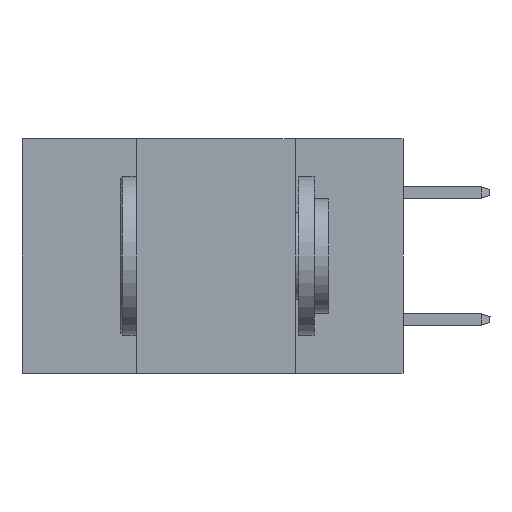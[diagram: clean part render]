
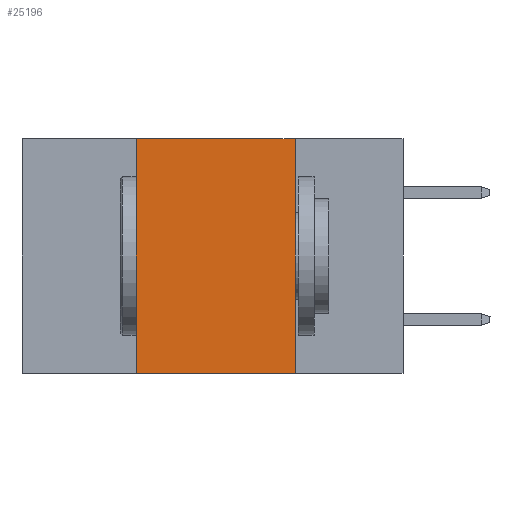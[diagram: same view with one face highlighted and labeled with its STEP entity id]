
A CAD part, left-side view. The second image highlights one B-rep face of the part: STEP entity #25196.
In plain terms, the highlighted planar face has unit normal (-1, 0, 0).
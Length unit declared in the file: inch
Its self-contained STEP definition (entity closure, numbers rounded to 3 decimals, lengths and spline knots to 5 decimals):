
#1171 = FACE_OUTER_BOUND ( 'NONE', #2502, .T. ) ;
#1726 = CARTESIAN_POINT ( 'NONE',  ( 0., 0.17, 0. ) ) ;
#1847 = DIRECTION ( 'NONE',  ( 0., -1., 0. ) ) ;
#2243 = VECTOR ( 'NONE', #7928, 39.37008 ) ;
#2502 = EDGE_LOOP ( 'NONE', ( #14716, #17885, #12714, #3835 ) ) ;
#3537 = VECTOR ( 'NONE', #1847, 39.37008 ) ;
#3766 = LINE ( 'NONE', #11602, #3537 ) ;
#3835 = ORIENTED_EDGE ( 'NONE', *, *, #11018, .T. ) ;
#4919 = VECTOR ( 'NONE', #22221, 39.37008 ) ;
#6716 = CARTESIAN_POINT ( 'NONE',  ( 0., 0.6, 0. ) ) ;
#7212 = CARTESIAN_POINT ( 'NONE',  ( 0., 0.42, -0.37 ) ) ;
#7320 = DIRECTION ( 'NONE',  ( 0., 0., -1. ) ) ;
#7928 = DIRECTION ( 'NONE',  ( 0., -1., 0. ) ) ;
#9028 = PLANE ( 'NONE',  #9874 ) ;
#9387 = CARTESIAN_POINT ( 'NONE',  ( 0., 0.17, 0. ) ) ;
#9874 = AXIS2_PLACEMENT_3D ( 'NONE', #6716, #16828, #24701 ) ;
#9923 = LINE ( 'NONE', #23919, #4919 ) ;
#11018 = EDGE_CURVE ( 'NONE', #14980, #21601, #23480, .T. ) ;
#11602 = CARTESIAN_POINT ( 'NONE',  ( 0., 0.6, 0. ) ) ;
#12053 = EDGE_CURVE ( 'NONE', #21912, #21601, #15380, .T. ) ;
#12714 = ORIENTED_EDGE ( 'NONE', *, *, #24049, .F. ) ;
#14544 = VECTOR ( 'NONE', #7320, 39.37008 ) ;
#14716 = ORIENTED_EDGE ( 'NONE', *, *, #12053, .F. ) ;
#14980 = VERTEX_POINT ( 'NONE', #7212 ) ;
#15158 = VERTEX_POINT ( 'NONE', #21239 ) ;
#15380 = LINE ( 'NONE', #9387, #14544 ) ;
#16338 = EDGE_CURVE ( 'NONE', #15158, #21912, #3766, .T. ) ;
#16828 = DIRECTION ( 'NONE',  ( 1., 0., 0. ) ) ;
#17885 = ORIENTED_EDGE ( 'NONE', *, *, #16338, .F. ) ;
#18018 = CARTESIAN_POINT ( 'NONE',  ( 0., 0.6, -0.37 ) ) ;
#20886 = CARTESIAN_POINT ( 'NONE',  ( 0., 0.17, -0.37 ) ) ;
#21239 = CARTESIAN_POINT ( 'NONE',  ( 0., 0.42, 0. ) ) ;
#21601 = VERTEX_POINT ( 'NONE', #20886 ) ;
#21912 = VERTEX_POINT ( 'NONE', #1726 ) ;
#22221 = DIRECTION ( 'NONE',  ( 0., 0., 1. ) ) ;
#23480 = LINE ( 'NONE', #18018, #2243 ) ;
#23919 = CARTESIAN_POINT ( 'NONE',  ( 0., 0.42, 0. ) ) ;
#24049 = EDGE_CURVE ( 'NONE', #14980, #15158, #9923, .T. ) ;
#24701 = DIRECTION ( 'NONE',  ( 0., 0., -1. ) ) ;
#25196 = ADVANCED_FACE ( 'NONE', ( #1171 ), #9028, .F. ) ;
